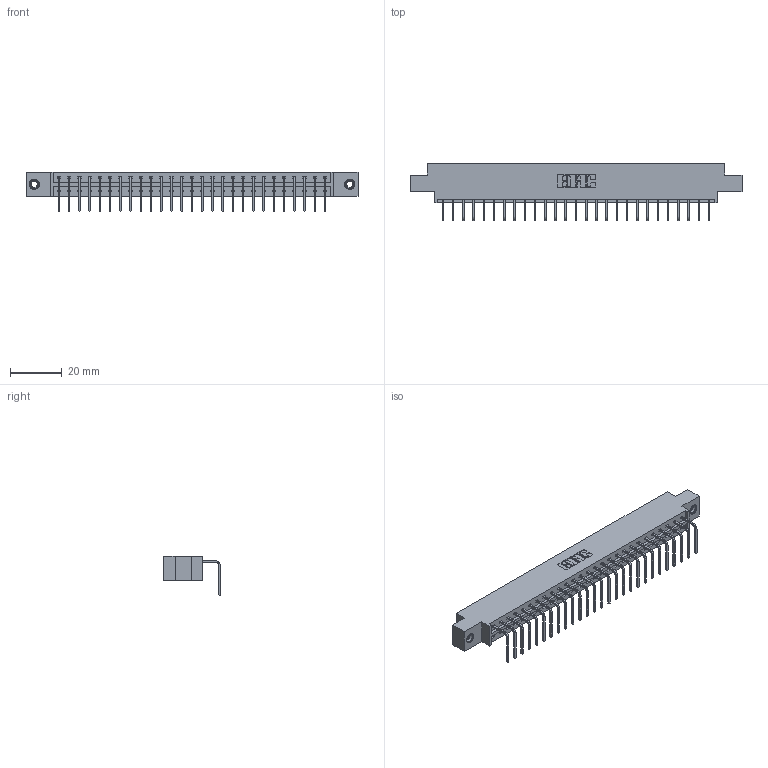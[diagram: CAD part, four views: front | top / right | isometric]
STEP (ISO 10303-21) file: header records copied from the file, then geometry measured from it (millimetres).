
FILE_DESCRIPTION (( 'STEP AP203' ), '1' );
FILE_NAME ('833-027-558-607.STEP', '2020-06-02T07:12:36', ( '' ), ( '' ), 'SwSTEP 2.0', 'SolidWorks 2020', '' );
FILE_SCHEMA (( 'CONFIG_CONTROL_DESIGN' ));
Length unit declared in the file: inch
Products named in the file (4): 345-250-001_345-250-005-103; 345-292-001_558 Tail - 2; 833-027-558-607; 833 Part_Offset - .156 Dia - TI
Assembly tree (30 placements, depth 2):
  833-027-558-607
    833 Part_Offset - .156 Dia - TI
    345-292-001_558 Tail - 2  x27
    345-250-001_345-250-005-103  x2
Bounding box: 128.52 x 22.17 x 15.37 mm (x, y, z)
Volume: 12652.8 mm3; surface area: 14379.1 mm2
Topology: 30 solids, 30 shells, 1798 faces, 5373 edges, 3538 vertices
Faces by surface type: plane 1294, cylinder 488, cone 12, torus 4
Entity records: 19848 total; most frequent: CARTESIAN_POINT 3410, ORIENTED_EDGE 3366, DIRECTION 2939, EDGE_CURVE 1683, LINE 1535, VECTOR 1535, VERTEX_POINT 1116, AXIS2_PLACEMENT_3D 702
